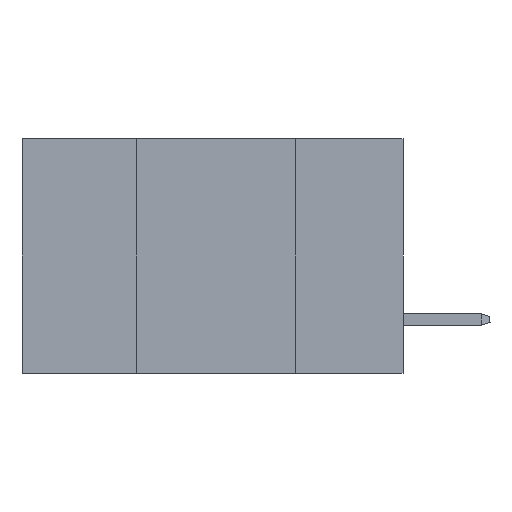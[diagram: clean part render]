
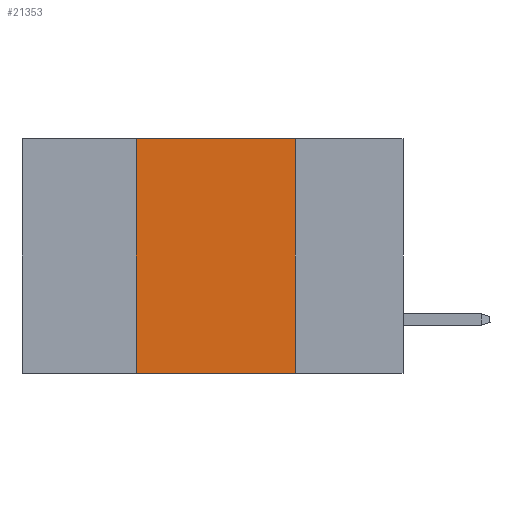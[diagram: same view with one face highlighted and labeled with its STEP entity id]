
A CAD part, left-side view. The second image highlights one B-rep face of the part: STEP entity #21353.
In plain terms, the highlighted planar face has unit normal (-1, 0, 0).
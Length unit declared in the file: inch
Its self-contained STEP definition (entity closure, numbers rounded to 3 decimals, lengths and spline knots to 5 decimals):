
#4087 = LINE ( 'NONE', #17713, #37392 ) ;
#4215 = LINE ( 'NONE', #17836, #36725 ) ;
#7300 = CARTESIAN_POINT ( 'NONE',  ( 0., 0.17, 0. ) ) ;
#8591 = VERTEX_POINT ( 'NONE', #18097 ) ;
#9195 = ORIENTED_EDGE ( 'NONE', *, *, #19794, .F. ) ;
#9985 = VERTEX_POINT ( 'NONE', #29756 ) ;
#11168 = EDGE_LOOP ( 'NONE', ( #18818, #9195, #36062, #23155 ) ) ;
#11486 = CARTESIAN_POINT ( 'NONE',  ( 0., 0.42, 0. ) ) ;
#13652 = CARTESIAN_POINT ( 'NONE',  ( 0., 0.6, 0. ) ) ;
#13784 = LINE ( 'NONE', #7300, #39878 ) ;
#15650 = VERTEX_POINT ( 'NONE', #16822 ) ;
#16822 = CARTESIAN_POINT ( 'NONE',  ( 0., 0.42, 0. ) ) ;
#17661 = DIRECTION ( 'NONE',  ( 0., 0., -1. ) ) ;
#17713 = CARTESIAN_POINT ( 'NONE',  ( 0., 0.6, 0. ) ) ;
#17836 = CARTESIAN_POINT ( 'NONE',  ( 0., 0.6, -0.37 ) ) ;
#18097 = CARTESIAN_POINT ( 'NONE',  ( 0., 0.17, 0. ) ) ;
#18818 = ORIENTED_EDGE ( 'NONE', *, *, #27157, .F. ) ;
#19794 = EDGE_CURVE ( 'NONE', #15650, #8591, #4087, .T. ) ;
#20239 = EDGE_CURVE ( 'NONE', #9985, #26425, #4215, .T. ) ;
#21353 = ADVANCED_FACE ( 'NONE', ( #34431 ), #24135, .F. ) ;
#23155 = ORIENTED_EDGE ( 'NONE', *, *, #20239, .T. ) ;
#24135 = PLANE ( 'NONE',  #37485 ) ;
#26425 = VERTEX_POINT ( 'NONE', #43487 ) ;
#27157 = EDGE_CURVE ( 'NONE', #8591, #26425, #13784, .T. ) ;
#29756 = CARTESIAN_POINT ( 'NONE',  ( 0., 0.42, -0.37 ) ) ;
#30770 = VECTOR ( 'NONE', #32053, 39.37008 ) ;
#30809 = DIRECTION ( 'NONE',  ( 0., -1., 0. ) ) ;
#31344 = DIRECTION ( 'NONE',  ( 0., -1., 0. ) ) ;
#32053 = DIRECTION ( 'NONE',  ( 0., 0., 1. ) ) ;
#34431 = FACE_OUTER_BOUND ( 'NONE', #11168, .T. ) ;
#34566 = DIRECTION ( 'NONE',  ( 0., 0., -1. ) ) ;
#36062 = ORIENTED_EDGE ( 'NONE', *, *, #36523, .F. ) ;
#36523 = EDGE_CURVE ( 'NONE', #9985, #15650, #38728, .T. ) ;
#36725 = VECTOR ( 'NONE', #30809, 39.37008 ) ;
#37341 = DIRECTION ( 'NONE',  ( 1., 0., 0. ) ) ;
#37392 = VECTOR ( 'NONE', #31344, 39.37008 ) ;
#37485 = AXIS2_PLACEMENT_3D ( 'NONE', #13652, #37341, #17661 ) ;
#38728 = LINE ( 'NONE', #11486, #30770 ) ;
#39878 = VECTOR ( 'NONE', #34566, 39.37008 ) ;
#43487 = CARTESIAN_POINT ( 'NONE',  ( 0., 0.17, -0.37 ) ) ;
